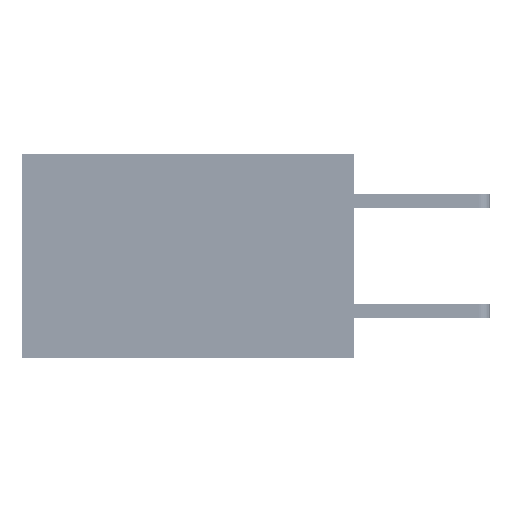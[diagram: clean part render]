
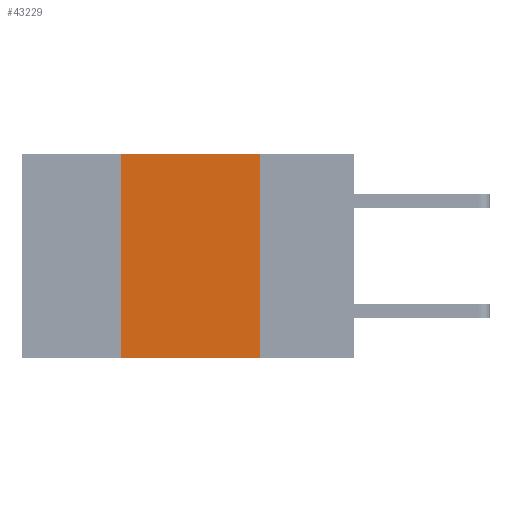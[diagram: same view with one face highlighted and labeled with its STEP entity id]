
A CAD part, left-side view. The second image highlights one B-rep face of the part: STEP entity #43229.
In plain terms, the highlighted planar face has unit normal (-1, 0, 0).
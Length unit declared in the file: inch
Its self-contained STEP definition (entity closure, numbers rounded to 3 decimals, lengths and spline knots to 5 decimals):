
#3692 = ORIENTED_EDGE ( 'NONE', *, *, #21978, .F. ) ;
#4067 = DIRECTION ( 'NONE',  ( 0., 0., 1. ) ) ;
#4150 = ORIENTED_EDGE ( 'NONE', *, *, #44760, .F. ) ;
#5463 = DIRECTION ( 'NONE',  ( 0., 0., -1. ) ) ;
#5625 = CARTESIAN_POINT ( 'NONE',  ( 0., 0.6, 0. ) ) ;
#7174 = CARTESIAN_POINT ( 'NONE',  ( 0., 0.17, 0. ) ) ;
#7730 = ORIENTED_EDGE ( 'NONE', *, *, #23111, .F. ) ;
#10276 = CARTESIAN_POINT ( 'NONE',  ( 0., 0.42, -0.37 ) ) ;
#11532 = VERTEX_POINT ( 'NONE', #10276 ) ;
#12410 = VECTOR ( 'NONE', #30384, 39.37008 ) ;
#13008 = VERTEX_POINT ( 'NONE', #47282 ) ;
#15354 = LINE ( 'NONE', #7174, #12410 ) ;
#16432 = EDGE_LOOP ( 'NONE', ( #7730, #4150, #3692, #26793 ) ) ;
#16939 = CARTESIAN_POINT ( 'NONE',  ( 0., 0.42, 0. ) ) ;
#17628 = AXIS2_PLACEMENT_3D ( 'NONE', #5625, #24126, #5463 ) ;
#18140 = CARTESIAN_POINT ( 'NONE',  ( 0., 0.6, -0.37 ) ) ;
#18685 = CARTESIAN_POINT ( 'NONE',  ( 0., 0.6, 0. ) ) ;
#20088 = PLANE ( 'NONE',  #17628 ) ;
#20984 = VERTEX_POINT ( 'NONE', #35976 ) ;
#21978 = EDGE_CURVE ( 'NONE', #11532, #24947, #39157, .T. ) ;
#22411 = DIRECTION ( 'NONE',  ( 0., -1., 0. ) ) ;
#23111 = EDGE_CURVE ( 'NONE', #13008, #20984, #15354, .T. ) ;
#23540 = CARTESIAN_POINT ( 'NONE',  ( 0., 0.42, 0. ) ) ;
#24126 = DIRECTION ( 'NONE',  ( 1., 0., 0. ) ) ;
#24947 = VERTEX_POINT ( 'NONE', #16939 ) ;
#26037 = VECTOR ( 'NONE', #22411, 39.37008 ) ;
#26793 = ORIENTED_EDGE ( 'NONE', *, *, #47100, .T. ) ;
#29303 = VECTOR ( 'NONE', #40826, 39.37008 ) ;
#30384 = DIRECTION ( 'NONE',  ( 0., 0., -1. ) ) ;
#35976 = CARTESIAN_POINT ( 'NONE',  ( 0., 0.17, -0.37 ) ) ;
#36307 = FACE_OUTER_BOUND ( 'NONE', #16432, .T. ) ;
#37973 = LINE ( 'NONE', #18140, #29303 ) ;
#39157 = LINE ( 'NONE', #23540, #42082 ) ;
#40826 = DIRECTION ( 'NONE',  ( 0., -1., 0. ) ) ;
#42082 = VECTOR ( 'NONE', #4067, 39.37008 ) ;
#43229 = ADVANCED_FACE ( 'NONE', ( #36307 ), #20088, .F. ) ;
#44013 = LINE ( 'NONE', #18685, #26037 ) ;
#44760 = EDGE_CURVE ( 'NONE', #24947, #13008, #44013, .T. ) ;
#47100 = EDGE_CURVE ( 'NONE', #11532, #20984, #37973, .T. ) ;
#47282 = CARTESIAN_POINT ( 'NONE',  ( 0., 0.17, 0. ) ) ;
